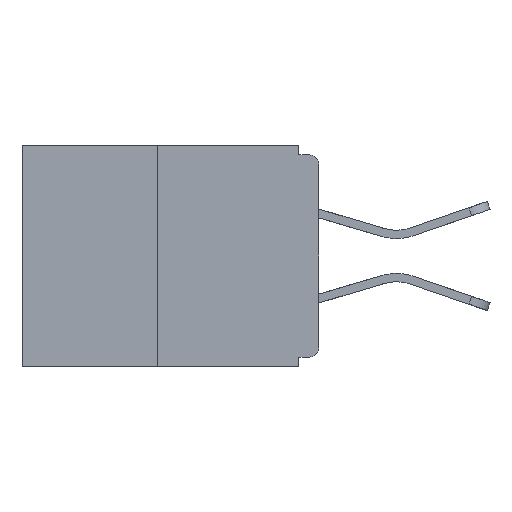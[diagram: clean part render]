
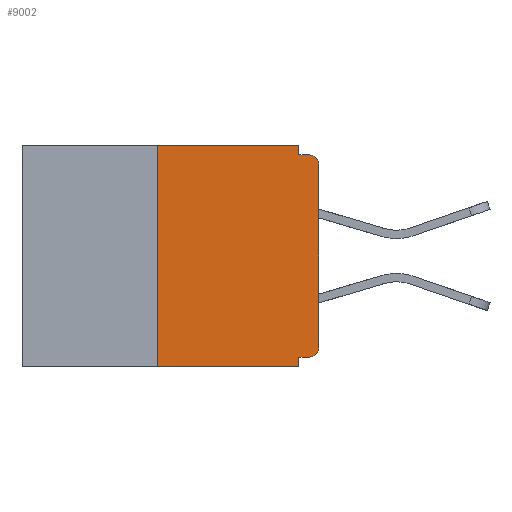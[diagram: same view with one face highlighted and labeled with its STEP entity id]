
A CAD part, left-side view. The second image highlights one B-rep face of the part: STEP entity #9002.
In plain terms, the highlighted planar face has unit normal (-1, 0, 0).
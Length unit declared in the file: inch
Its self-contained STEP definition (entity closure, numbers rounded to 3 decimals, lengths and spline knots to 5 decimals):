
#54 = DIRECTION ( 'NONE',  ( 0., 0., 1. ) ) ;
#204 = VERTEX_POINT ( 'NONE', #963 ) ;
#336 = DIRECTION ( 'NONE',  ( 0., 0., -1. ) ) ;
#353 = DIRECTION ( 'NONE',  ( 0., 0., -1. ) ) ;
#354 = LINE ( 'NONE', #12078, #10928 ) ;
#370 = VECTOR ( 'NONE', #435, 39.37008 ) ;
#435 = DIRECTION ( 'NONE',  ( 0., 1., 0. ) ) ;
#465 = CARTESIAN_POINT ( 'NONE',  ( 0., 0.46, 0. ) ) ;
#963 = CARTESIAN_POINT ( 'NONE',  ( 0., 0., -0.313 ) ) ;
#970 = ORIENTED_EDGE ( 'NONE', *, *, #5044, .F. ) ;
#1044 = VERTEX_POINT ( 'NONE', #9786 ) ;
#1086 = DIRECTION ( 'NONE',  ( -1., 0., 0. ) ) ;
#1152 = VECTOR ( 'NONE', #1382, 39.37008 ) ;
#1382 = DIRECTION ( 'NONE',  ( 0., 0., -1. ) ) ;
#1627 = EDGE_CURVE ( 'NONE', #1044, #6088, #11918, .T. ) ;
#2202 = CARTESIAN_POINT ( 'NONE',  ( 0., 0.25, 0. ) ) ;
#2204 = EDGE_CURVE ( 'NONE', #2313, #4208, #354, .T. ) ;
#2232 = EDGE_CURVE ( 'NONE', #6384, #10095, #4182, .T. ) ;
#2313 = VERTEX_POINT ( 'NONE', #4159 ) ;
#2355 = AXIS2_PLACEMENT_3D ( 'NONE', #10716, #1086, #8599 ) ;
#2792 = PLANE ( 'NONE',  #10977 ) ;
#2836 = VECTOR ( 'NONE', #11721, 39.37008 ) ;
#2963 = CARTESIAN_POINT ( 'NONE',  ( 0., 0.031, -0.015 ) ) ;
#3334 = EDGE_CURVE ( 'NONE', #204, #9031, #4147, .T. ) ;
#3505 = CARTESIAN_POINT ( 'NONE',  ( 0., 0.031, -0.343 ) ) ;
#3574 = DIRECTION ( 'NONE',  ( 1., 0., 0. ) ) ;
#3808 = CARTESIAN_POINT ( 'NONE',  ( 0., 0., -0.03 ) ) ;
#3952 = CARTESIAN_POINT ( 'NONE',  ( 0., 0.031, -0.328 ) ) ;
#3980 = CARTESIAN_POINT ( 'NONE',  ( 0., 0.015, -0.03 ) ) ;
#4117 = ORIENTED_EDGE ( 'NONE', *, *, #2204, .T. ) ;
#4147 = LINE ( 'NONE', #6489, #2836 ) ;
#4159 = CARTESIAN_POINT ( 'NONE',  ( 0., 0.25, -0.343 ) ) ;
#4182 = LINE ( 'NONE', #465, #7476 ) ;
#4208 = VERTEX_POINT ( 'NONE', #6595 ) ;
#4545 = CARTESIAN_POINT ( 'NONE',  ( 0., 0., -0.328 ) ) ;
#4548 = VECTOR ( 'NONE', #6206, 39.37008 ) ;
#5001 = CARTESIAN_POINT ( 'NONE',  ( 0., 0., -0.015 ) ) ;
#5044 = EDGE_CURVE ( 'NONE', #2313, #6384, #9274, .T. ) ;
#5146 = VECTOR ( 'NONE', #54, 39.37008 ) ;
#5771 = DIRECTION ( 'NONE',  ( 0., -1., 0. ) ) ;
#5845 = CIRCLE ( 'NONE', #10305, 0.015 ) ;
#5930 = LINE ( 'NONE', #3505, #10860 ) ;
#6088 = VERTEX_POINT ( 'NONE', #3952 ) ;
#6206 = DIRECTION ( 'NONE',  ( 0., -1., 0. ) ) ;
#6376 = EDGE_LOOP ( 'NONE', ( #12246, #970, #4117, #10777, #9098, #11041, #10141, #12937, #7090, #11252 ) ) ;
#6384 = VERTEX_POINT ( 'NONE', #6515 ) ;
#6489 = CARTESIAN_POINT ( 'NONE',  ( 0., 0., 0. ) ) ;
#6515 = CARTESIAN_POINT ( 'NONE',  ( 0., 0.25, 0. ) ) ;
#6595 = CARTESIAN_POINT ( 'NONE',  ( 0., 0.031, -0.343 ) ) ;
#6864 = VERTEX_POINT ( 'NONE', #9473 ) ;
#6976 = CARTESIAN_POINT ( 'NONE',  ( 0., 0.46, 0. ) ) ;
#7090 = ORIENTED_EDGE ( 'NONE', *, *, #8355, .F. ) ;
#7444 = LINE ( 'NONE', #8936, #1152 ) ;
#7476 = VECTOR ( 'NONE', #8856, 39.37008 ) ;
#8128 = DIRECTION ( 'NONE',  ( -1., 0., 0. ) ) ;
#8355 = EDGE_CURVE ( 'NONE', #12227, #6864, #12609, .T. ) ;
#8599 = DIRECTION ( 'NONE',  ( 0., 0., -1. ) ) ;
#8856 = DIRECTION ( 'NONE',  ( 0., -1., 0. ) ) ;
#8936 = CARTESIAN_POINT ( 'NONE',  ( 0., 0.031, 0. ) ) ;
#8944 = CARTESIAN_POINT ( 'NONE',  ( 0., 0.031, 0. ) ) ;
#9002 = ADVANCED_FACE ( 'NONE', ( #12281 ), #2792, .F. ) ;
#9031 = VERTEX_POINT ( 'NONE', #3808 ) ;
#9098 = ORIENTED_EDGE ( 'NONE', *, *, #1627, .F. ) ;
#9264 = DIRECTION ( 'NONE',  ( 0., 0., -1. ) ) ;
#9274 = LINE ( 'NONE', #2202, #5146 ) ;
#9473 = CARTESIAN_POINT ( 'NONE',  ( 0., 0.015, -0.015 ) ) ;
#9786 = CARTESIAN_POINT ( 'NONE',  ( 0., 0.015, -0.328 ) ) ;
#9816 = EDGE_CURVE ( 'NONE', #6088, #4208, #5930, .T. ) ;
#10095 = VERTEX_POINT ( 'NONE', #8944 ) ;
#10141 = ORIENTED_EDGE ( 'NONE', *, *, #3334, .T. ) ;
#10305 = AXIS2_PLACEMENT_3D ( 'NONE', #3980, #8128, #9264 ) ;
#10716 = CARTESIAN_POINT ( 'NONE',  ( 0., 0.015, -0.313 ) ) ;
#10777 = ORIENTED_EDGE ( 'NONE', *, *, #9816, .F. ) ;
#10832 = EDGE_CURVE ( 'NONE', #1044, #204, #12108, .T. ) ;
#10860 = VECTOR ( 'NONE', #336, 39.37008 ) ;
#10928 = VECTOR ( 'NONE', #5771, 39.37008 ) ;
#10977 = AXIS2_PLACEMENT_3D ( 'NONE', #6976, #3574, #353 ) ;
#11041 = ORIENTED_EDGE ( 'NONE', *, *, #10832, .T. ) ;
#11155 = EDGE_CURVE ( 'NONE', #9031, #6864, #5845, .T. ) ;
#11252 = ORIENTED_EDGE ( 'NONE', *, *, #13281, .F. ) ;
#11721 = DIRECTION ( 'NONE',  ( 0., 0., 1. ) ) ;
#11918 = LINE ( 'NONE', #4545, #370 ) ;
#12078 = CARTESIAN_POINT ( 'NONE',  ( 0., 0.46, -0.343 ) ) ;
#12108 = CIRCLE ( 'NONE', #2355, 0.015 ) ;
#12227 = VERTEX_POINT ( 'NONE', #2963 ) ;
#12246 = ORIENTED_EDGE ( 'NONE', *, *, #2232, .F. ) ;
#12281 = FACE_OUTER_BOUND ( 'NONE', #6376, .T. ) ;
#12609 = LINE ( 'NONE', #5001, #4548 ) ;
#12937 = ORIENTED_EDGE ( 'NONE', *, *, #11155, .T. ) ;
#13281 = EDGE_CURVE ( 'NONE', #10095, #12227, #7444, .T. ) ;
